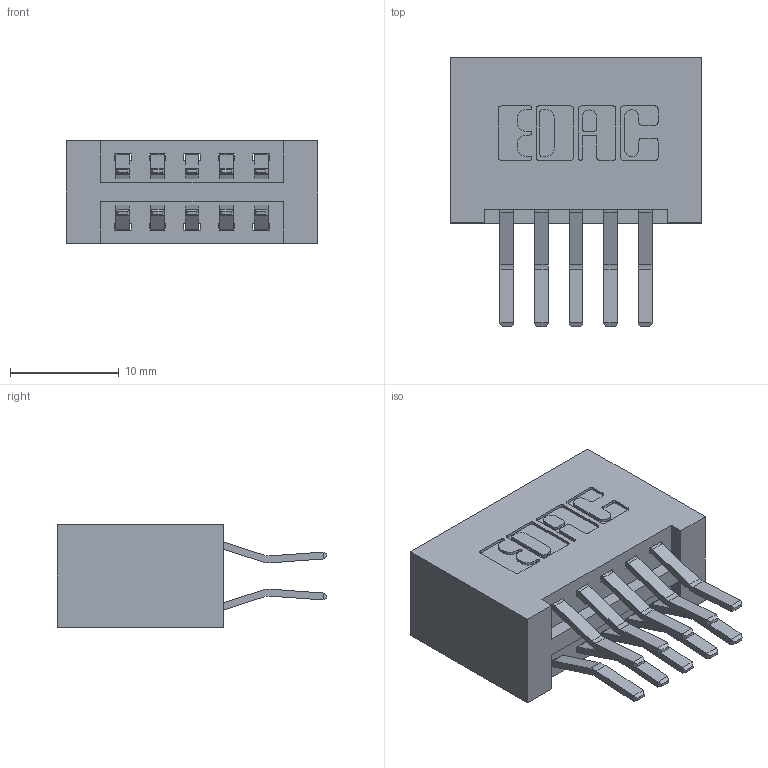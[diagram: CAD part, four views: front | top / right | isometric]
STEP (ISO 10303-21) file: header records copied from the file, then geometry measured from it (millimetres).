
FILE_DESCRIPTION (( 'STEP AP203' ), '1' );
FILE_NAME ('346-010-560-201.STEP', '2018-08-17T08:11:30', ( '' ), ( '' ), 'SwSTEP 2.0', 'SolidWorks 2016', '' );
FILE_SCHEMA (( 'CONFIG_CONTROL_DESIGN' ));
Length unit declared in the file: inch
Products named in the file (3): 346 Part_No Mounting Lugs; 345-292-001_560 Tail; 346-010-560-201
Assembly tree (11 placements, depth 2):
  346-010-560-201
    346 Part_No Mounting Lugs
    345-292-001_560 Tail  x10
Bounding box: 23.11 x 24.78 x 9.4 mm (x, y, z)
Volume: 2605.4 mm3; surface area: 3337.8 mm2
Topology: 11 solids, 11 shells, 654 faces, 1915 edges, 1262 vertices
Faces by surface type: plane 422, cylinder 232
Entity records: 8055 total; most frequent: CARTESIAN_POINT 1376, ORIENTED_EDGE 1310, DIRECTION 1263, EDGE_CURVE 655, VECTOR 507, LINE 507, VERTEX_POINT 434, AXIS2_PLACEMENT_3D 378
